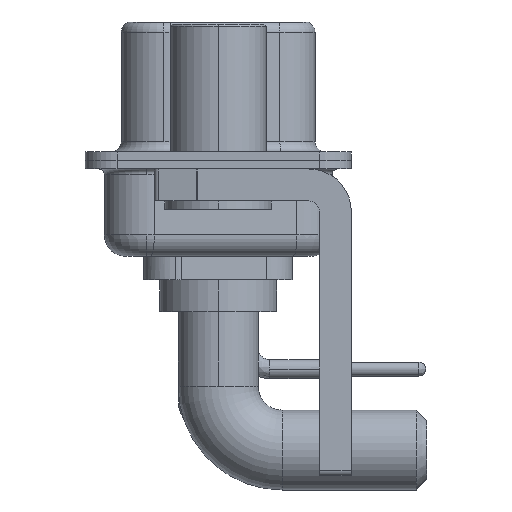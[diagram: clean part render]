
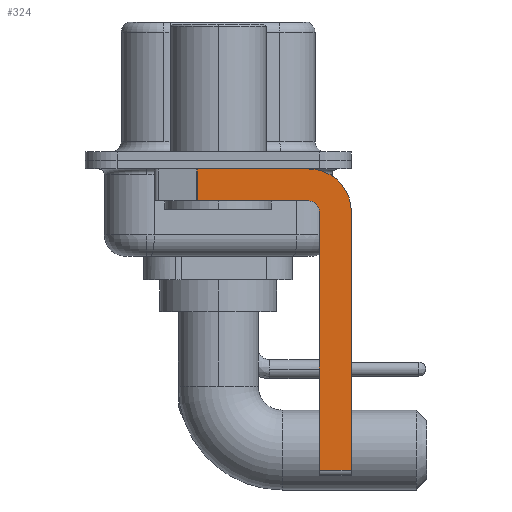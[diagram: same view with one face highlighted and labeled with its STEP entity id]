
A CAD part, left-side view. The second image highlights one B-rep face of the part: STEP entity #324.
In plain terms, the highlighted planar face has unit normal (-1, 0, 0).
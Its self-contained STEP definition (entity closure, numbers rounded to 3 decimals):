
#138 = DIRECTION ( 'NONE',  ( 0., 1., 0. ) ) ;
#324 = ADVANCED_FACE ( 'NONE', ( #22146 ), #437, .F. ) ;
#344 = ORIENTED_EDGE ( 'NONE', *, *, #4182, .T. ) ;
#437 = PLANE ( 'NONE',  #3447 ) ;
#543 = CARTESIAN_POINT ( 'NONE',  ( -2.9, -4.75, -14.55 ) ) ;
#639 = VECTOR ( 'NONE', #19345, 1000. ) ;
#645 = CARTESIAN_POINT ( 'NONE',  ( -2.9, 0.978, -0.4 ) ) ;
#703 = ORIENTED_EDGE ( 'NONE', *, *, #18798, .F. ) ;
#1108 = DIRECTION ( 'NONE',  ( 0., 0., -1. ) ) ;
#1746 = VERTEX_POINT ( 'NONE', #645 ) ;
#2157 = CARTESIAN_POINT ( 'NONE',  ( -2.9, -6.25, -2.4 ) ) ;
#2238 = ORIENTED_EDGE ( 'NONE', *, *, #17435, .F. ) ;
#2601 = LINE ( 'NONE', #2157, #4655 ) ;
#2883 = VECTOR ( 'NONE', #1108, 1000. ) ;
#2899 = CARTESIAN_POINT ( 'NONE',  ( -2.9, 0.978, -1.9 ) ) ;
#3148 = DIRECTION ( 'NONE',  ( 0., -1., 0. ) ) ;
#3319 = CARTESIAN_POINT ( 'NONE',  ( -2.9, 0.978, -1.9 ) ) ;
#3447 = AXIS2_PLACEMENT_3D ( 'NONE', #11254, #5785, #13019 ) ;
#3728 = VERTEX_POINT ( 'NONE', #21476 ) ;
#3810 = AXIS2_PLACEMENT_3D ( 'NONE', #4509, #17428, #22764 ) ;
#4182 = EDGE_CURVE ( 'NONE', #1746, #19109, #17257, .T. ) ;
#4315 = CARTESIAN_POINT ( 'NONE',  ( -2.9, -4.25, -2.4 ) ) ;
#4509 = CARTESIAN_POINT ( 'NONE',  ( -2.9, -4.25, -2.4 ) ) ;
#4655 = VECTOR ( 'NONE', #9042, 1000. ) ;
#4825 = LINE ( 'NONE', #8507, #7101 ) ;
#5785 = DIRECTION ( 'NONE',  ( 1., 0., 0. ) ) ;
#6257 = CIRCLE ( 'NONE', #16848, 2. ) ;
#6664 = ORIENTED_EDGE ( 'NONE', *, *, #12709, .F. ) ;
#7030 = VECTOR ( 'NONE', #138, 1000. ) ;
#7101 = VECTOR ( 'NONE', #3148, 1000. ) ;
#8229 = CARTESIAN_POINT ( 'NONE',  ( -2.9, -4.25, -14.55 ) ) ;
#8507 = CARTESIAN_POINT ( 'NONE',  ( -2.9, 3., -0.4 ) ) ;
#9000 = VECTOR ( 'NONE', #13020, 1000. ) ;
#9042 = DIRECTION ( 'NONE',  ( 0., 0., -1. ) ) ;
#11254 = CARTESIAN_POINT ( 'NONE',  ( -2.9, -4.25, -2.4 ) ) ;
#11538 = VERTEX_POINT ( 'NONE', #21963 ) ;
#11757 = LINE ( 'NONE', #8229, #639 ) ;
#12256 = ORIENTED_EDGE ( 'NONE', *, *, #18293, .F. ) ;
#12493 = EDGE_CURVE ( 'NONE', #16529, #19529, #18484, .T. ) ;
#12709 = EDGE_CURVE ( 'NONE', #1746, #11538, #4825, .T. ) ;
#12854 = DIRECTION ( 'NONE',  ( 1., 0., 0. ) ) ;
#13019 = DIRECTION ( 'NONE',  ( 0., 0., -1. ) ) ;
#13020 = DIRECTION ( 'NONE',  ( 0., 0., 1. ) ) ;
#13068 = LINE ( 'NONE', #16394, #7030 ) ;
#13757 = EDGE_CURVE ( 'NONE', #16529, #3728, #11757, .T. ) ;
#14754 = DIRECTION ( 'NONE',  ( 0., 0., -1. ) ) ;
#14787 = CIRCLE ( 'NONE', #3810, 0.5 ) ;
#14923 = CARTESIAN_POINT ( 'NONE',  ( -2.9, -4.75, -14.8 ) ) ;
#15115 = EDGE_CURVE ( 'NONE', #19529, #19056, #14787, .T. ) ;
#15953 = ORIENTED_EDGE ( 'NONE', *, *, #13757, .T. ) ;
#16394 = CARTESIAN_POINT ( 'NONE',  ( -2.9, -4.25, -1.9 ) ) ;
#16529 = VERTEX_POINT ( 'NONE', #543 ) ;
#16848 = AXIS2_PLACEMENT_3D ( 'NONE', #4315, #12854, #14754 ) ;
#17202 = ORIENTED_EDGE ( 'NONE', *, *, #15115, .F. ) ;
#17257 = LINE ( 'NONE', #2899, #2883 ) ;
#17283 = ORIENTED_EDGE ( 'NONE', *, *, #12493, .F. ) ;
#17428 = DIRECTION ( 'NONE',  ( -1., 0., 0. ) ) ;
#17435 = EDGE_CURVE ( 'NONE', #22262, #3728, #2601, .T. ) ;
#17530 = CARTESIAN_POINT ( 'NONE',  ( -2.9, -4.75, -2.4 ) ) ;
#18293 = EDGE_CURVE ( 'NONE', #11538, #22262, #6257, .T. ) ;
#18484 = LINE ( 'NONE', #14923, #9000 ) ;
#18798 = EDGE_CURVE ( 'NONE', #19056, #19109, #13068, .T. ) ;
#19056 = VERTEX_POINT ( 'NONE', #19803 ) ;
#19109 = VERTEX_POINT ( 'NONE', #3319 ) ;
#19345 = DIRECTION ( 'NONE',  ( 0., -1., 0. ) ) ;
#19529 = VERTEX_POINT ( 'NONE', #17530 ) ;
#19549 = EDGE_LOOP ( 'NONE', ( #6664, #344, #703, #17202, #17283, #15953, #2238, #12256 ) ) ;
#19803 = CARTESIAN_POINT ( 'NONE',  ( -2.9, -4.25, -1.9 ) ) ;
#19856 = CARTESIAN_POINT ( 'NONE',  ( -2.9, -6.25, -2.4 ) ) ;
#21476 = CARTESIAN_POINT ( 'NONE',  ( -2.9, -6.25, -14.55 ) ) ;
#21963 = CARTESIAN_POINT ( 'NONE',  ( -2.9, -4.25, -0.4 ) ) ;
#22146 = FACE_OUTER_BOUND ( 'NONE', #19549, .T. ) ;
#22262 = VERTEX_POINT ( 'NONE', #19856 ) ;
#22764 = DIRECTION ( 'NONE',  ( 0., 0., 1. ) ) ;
